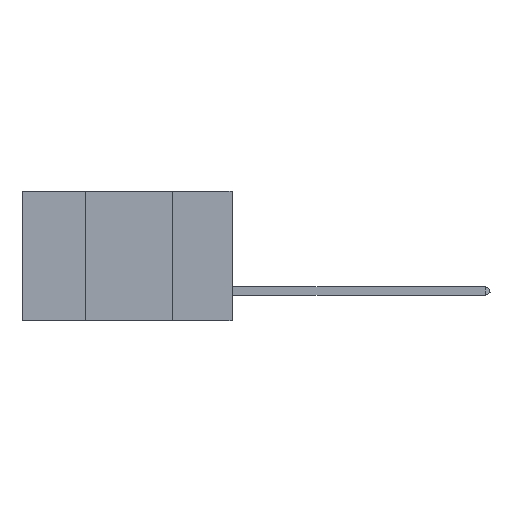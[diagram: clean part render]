
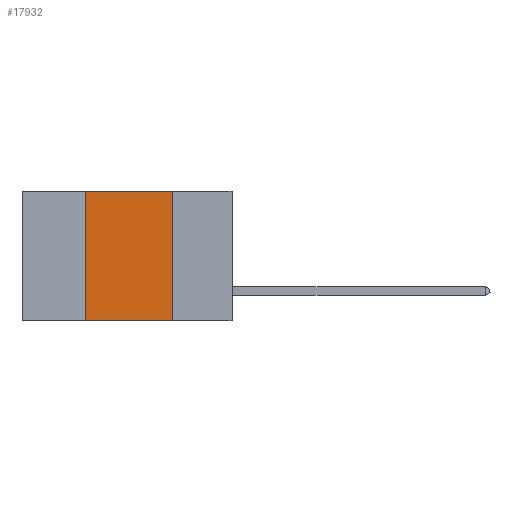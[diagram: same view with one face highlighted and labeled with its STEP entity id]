
A CAD part, left-side view. The second image highlights one B-rep face of the part: STEP entity #17932.
In plain terms, the highlighted planar face has unit normal (-1, 0, 0).
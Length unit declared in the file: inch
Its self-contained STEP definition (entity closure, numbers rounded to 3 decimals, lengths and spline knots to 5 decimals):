
#457 = VECTOR ( 'NONE', #19466, 39.37008 ) ;
#1109 = VERTEX_POINT ( 'NONE', #1863 ) ;
#1863 = CARTESIAN_POINT ( 'NONE',  ( 0., 0.17, -0.37 ) ) ;
#3040 = LINE ( 'NONE', #14112, #13220 ) ;
#3325 = EDGE_CURVE ( 'NONE', #14679, #14537, #19785, .T. ) ;
#3818 = DIRECTION ( 'NONE',  ( 0., 0., 1. ) ) ;
#4065 = CARTESIAN_POINT ( 'NONE',  ( 0., 0.17, 0. ) ) ;
#4339 = DIRECTION ( 'NONE',  ( 1., 0., 0. ) ) ;
#4721 = CARTESIAN_POINT ( 'NONE',  ( 0., 0.17, 0. ) ) ;
#5561 = VECTOR ( 'NONE', #3818, 39.37008 ) ;
#5720 = CARTESIAN_POINT ( 'NONE',  ( 0., 0.6, 0. ) ) ;
#6005 = CARTESIAN_POINT ( 'NONE',  ( 0., 0.42, 0. ) ) ;
#7677 = LINE ( 'NONE', #4721, #457 ) ;
#8026 = VERTEX_POINT ( 'NONE', #4065 ) ;
#9013 = ORIENTED_EDGE ( 'NONE', *, *, #14609, .F. ) ;
#9454 = ORIENTED_EDGE ( 'NONE', *, *, #3325, .F. ) ;
#9474 = FACE_OUTER_BOUND ( 'NONE', #21057, .T. ) ;
#12715 = ORIENTED_EDGE ( 'NONE', *, *, #24360, .T. ) ;
#12781 = PLANE ( 'NONE',  #22114 ) ;
#12946 = CARTESIAN_POINT ( 'NONE',  ( 0., 0.6, 0. ) ) ;
#13220 = VECTOR ( 'NONE', #16153, 39.37008 ) ;
#13350 = LINE ( 'NONE', #5720, #16020 ) ;
#14112 = CARTESIAN_POINT ( 'NONE',  ( 0., 0.6, -0.37 ) ) ;
#14537 = VERTEX_POINT ( 'NONE', #23745 ) ;
#14609 = EDGE_CURVE ( 'NONE', #8026, #1109, #7677, .T. ) ;
#14679 = VERTEX_POINT ( 'NONE', #22075 ) ;
#15177 = DIRECTION ( 'NONE',  ( 0., 0., -1. ) ) ;
#16020 = VECTOR ( 'NONE', #27016, 39.37008 ) ;
#16153 = DIRECTION ( 'NONE',  ( 0., -1., 0. ) ) ;
#17932 = ADVANCED_FACE ( 'NONE', ( #9474 ), #12781, .F. ) ;
#19466 = DIRECTION ( 'NONE',  ( 0., 0., -1. ) ) ;
#19785 = LINE ( 'NONE', #6005, #5561 ) ;
#20708 = ORIENTED_EDGE ( 'NONE', *, *, #27126, .F. ) ;
#21057 = EDGE_LOOP ( 'NONE', ( #9013, #20708, #9454, #12715 ) ) ;
#22075 = CARTESIAN_POINT ( 'NONE',  ( 0., 0.42, -0.37 ) ) ;
#22114 = AXIS2_PLACEMENT_3D ( 'NONE', #12946, #4339, #15177 ) ;
#23745 = CARTESIAN_POINT ( 'NONE',  ( 0., 0.42, 0. ) ) ;
#24360 = EDGE_CURVE ( 'NONE', #14679, #1109, #3040, .T. ) ;
#27016 = DIRECTION ( 'NONE',  ( 0., -1., 0. ) ) ;
#27126 = EDGE_CURVE ( 'NONE', #14537, #8026, #13350, .T. ) ;
